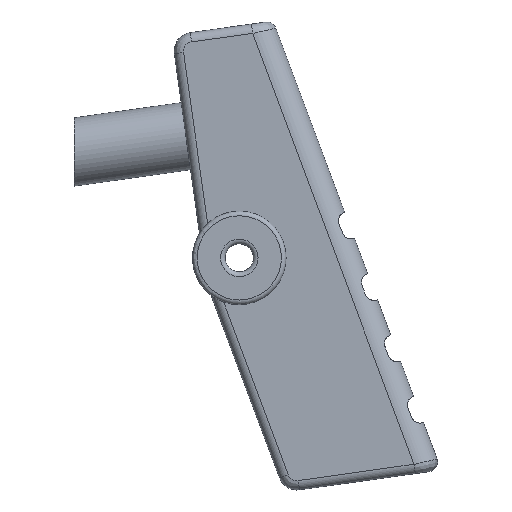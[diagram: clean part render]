
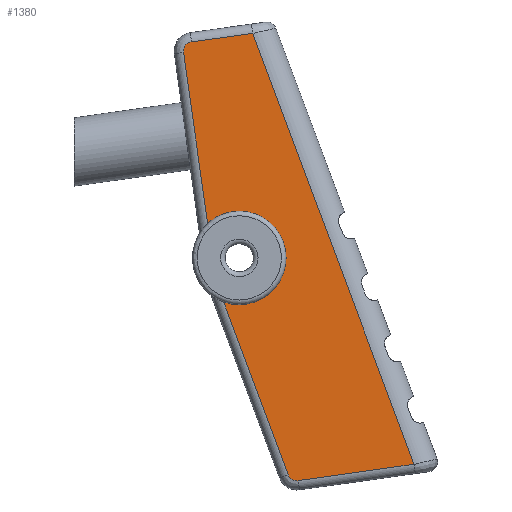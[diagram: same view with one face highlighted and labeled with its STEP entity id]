
A CAD part, left-side view. The second image highlights one B-rep face of the part: STEP entity #1380.
In plain terms, the highlighted planar face has unit normal (-1, 0, 0).
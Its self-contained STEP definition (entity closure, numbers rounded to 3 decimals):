
#84=CIRCLE('',#1506,5.);
#86=CIRCLE('',#1508,5.);
#88=CIRCLE('',#1512,1.);
#89=CIRCLE('',#1513,1.);
#146=PLANE('',#1511);
#182=FACE_OUTER_BOUND('',#272,.T.);
#272=EDGE_LOOP('',(#975,#976,#977,#978,#979,#980,#981,#982,#983));
#363=LINE('',#2233,#459);
#364=LINE('',#2237,#460);
#365=LINE('',#2239,#461);
#366=LINE('',#2241,#462);
#367=LINE('',#2244,#463);
#459=VECTOR('',#1741,10.);
#460=VECTOR('',#1744,10.);
#461=VECTOR('',#1745,10.);
#462=VECTOR('',#1746,10.);
#463=VECTOR('',#1749,10.);
#587=VERTEX_POINT('',#2192);
#588=VERTEX_POINT('',#2193);
#589=VERTEX_POINT('',#2195);
#594=VERTEX_POINT('',#2232);
#595=VERTEX_POINT('',#2234);
#596=VERTEX_POINT('',#2236);
#597=VERTEX_POINT('',#2238);
#598=VERTEX_POINT('',#2240);
#599=VERTEX_POINT('',#2242);
#728=EDGE_CURVE('',#589,#588,#84,.T.);
#730=EDGE_CURVE('',#587,#589,#86,.T.);
#736=EDGE_CURVE('',#594,#588,#363,.T.);
#737=EDGE_CURVE('',#595,#594,#88,.T.);
#738=EDGE_CURVE('',#596,#595,#364,.T.);
#739=EDGE_CURVE('',#597,#596,#365,.T.);
#740=EDGE_CURVE('',#598,#597,#366,.T.);
#741=EDGE_CURVE('',#599,#598,#89,.T.);
#742=EDGE_CURVE('',#587,#599,#367,.T.);
#975=ORIENTED_EDGE('',*,*,#730,.T.);
#976=ORIENTED_EDGE('',*,*,#728,.T.);
#977=ORIENTED_EDGE('',*,*,#736,.F.);
#978=ORIENTED_EDGE('',*,*,#737,.F.);
#979=ORIENTED_EDGE('',*,*,#738,.F.);
#980=ORIENTED_EDGE('',*,*,#739,.F.);
#981=ORIENTED_EDGE('',*,*,#740,.F.);
#982=ORIENTED_EDGE('',*,*,#741,.F.);
#983=ORIENTED_EDGE('',*,*,#742,.F.);
#1380=ADVANCED_FACE('',(#182),#146,.T.);
#1506=AXIS2_PLACEMENT_3D('',#2196,#1727,#1728);
#1508=AXIS2_PLACEMENT_3D('',#2198,#1731,#1732);
#1511=AXIS2_PLACEMENT_3D('',#2231,#1739,#1740);
#1512=AXIS2_PLACEMENT_3D('',#2235,#1742,#1743);
#1513=AXIS2_PLACEMENT_3D('',#2243,#1747,#1748);
#1727=DIRECTION('center_axis',(1.,0.,0.));
#1728=DIRECTION('ref_axis',(0.,-1.,0.));
#1731=DIRECTION('center_axis',(1.,0.,0.));
#1732=DIRECTION('ref_axis',(0.,-1.,0.));
#1739=DIRECTION('center_axis',(-1.,0.,0.));
#1740=DIRECTION('ref_axis',(0.,0.139,0.99));
#1741=DIRECTION('',(0.,0.351,0.936));
#1742=DIRECTION('center_axis',(1.,0.,0.));
#1743=DIRECTION('ref_axis',(0.,0.511,-0.86));
#1744=DIRECTION('',(0.,0.99,-0.139));
#1745=DIRECTION('',(0.,-0.351,-0.936));
#1746=DIRECTION('',(0.,-0.99,0.139));
#1747=DIRECTION('center_axis',(1.,0.,0.));
#1748=DIRECTION('ref_axis',(0.,0.799,0.602));
#1749=DIRECTION('',(0.,0.139,0.99));
#2192=CARTESIAN_POINT('',(-10.223,-3.557,111.618));
#2193=CARTESIAN_POINT('',(-10.223,-5.268,103.228));
#2195=CARTESIAN_POINT('',(-10.223,-6.943,112.939));
#2196=CARTESIAN_POINT('Origin',(-10.223,-6.943,107.939));
#2198=CARTESIAN_POINT('Origin',(-10.223,-6.943,107.939));
#2231=CARTESIAN_POINT('Origin',(-10.223,-13.451,105.886));
#2232=CARTESIAN_POINT('',(-10.223,-12.174,84.786));
#2233=CARTESIAN_POINT('',(-10.223,-8.927,93.456));
#2234=CARTESIAN_POINT('',(-10.223,-13.249,84.146));
#2235=CARTESIAN_POINT('Origin',(-10.223,-13.11,85.136));
#2236=CARTESIAN_POINT('',(-10.223,-25.618,85.884));
#2237=CARTESIAN_POINT('',(-10.223,-11.492,83.899));
#2238=CARTESIAN_POINT('',(-10.223,-8.375,131.933));
#2239=CARTESIAN_POINT('',(-10.223,-21.785,96.122));
#2240=CARTESIAN_POINT('',(-10.223,-1.84,131.014));
#2241=CARTESIAN_POINT('',(-10.223,-9.763,132.128));
#2242=CARTESIAN_POINT('',(-10.223,-0.989,129.885));
#2243=CARTESIAN_POINT('Origin',(-10.223,-1.98,130.024));
#2244=CARTESIAN_POINT('',(-10.223,-2.973,115.774));
